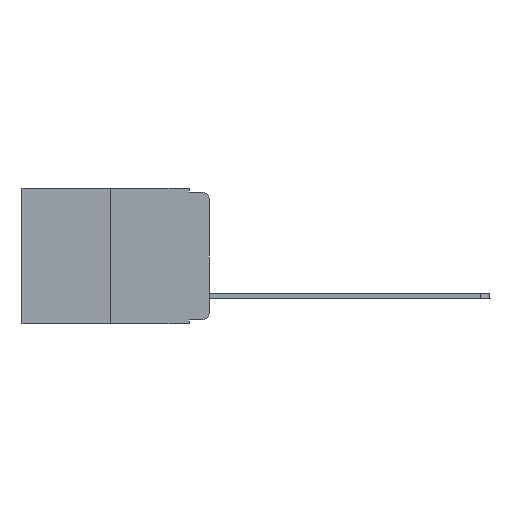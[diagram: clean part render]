
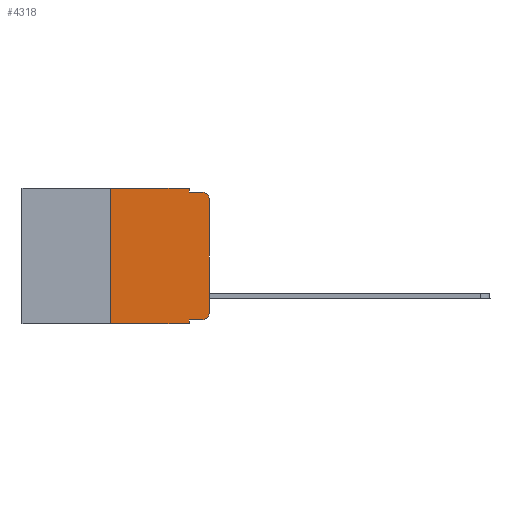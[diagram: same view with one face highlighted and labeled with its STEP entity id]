
A CAD part, left-side view. The second image highlights one B-rep face of the part: STEP entity #4318.
In plain terms, the highlighted planar face has unit normal (-1, 0, 0).
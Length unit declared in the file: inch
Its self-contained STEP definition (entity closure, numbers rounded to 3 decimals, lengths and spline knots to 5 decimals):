
#48 = CARTESIAN_POINT ( 'NONE',  ( 0., 0., 0. ) ) ;
#439 = CARTESIAN_POINT ( 'NONE',  ( 0., 0.051, -0.343 ) ) ;
#1055 = ORIENTED_EDGE ( 'NONE', *, *, #1664, .T. ) ;
#1243 = CARTESIAN_POINT ( 'NONE',  ( 0., 0.051, -0.333 ) ) ;
#1499 = DIRECTION ( 'NONE',  ( -1., 0., 0. ) ) ;
#1664 = EDGE_CURVE ( 'NONE', #16182, #15364, #4769, .T. ) ;
#1718 = ORIENTED_EDGE ( 'NONE', *, *, #10198, .T. ) ;
#1774 = VERTEX_POINT ( 'NONE', #4025 ) ;
#2221 = DIRECTION ( 'NONE',  ( -1., 0., 0. ) ) ;
#2306 = LINE ( 'NONE', #11576, #17521 ) ;
#2765 = LINE ( 'NONE', #4260, #10580 ) ;
#2769 = DIRECTION ( 'NONE',  ( 0., -1., 0. ) ) ;
#2883 = DIRECTION ( 'NONE',  ( 0., -1., 0. ) ) ;
#3223 = CARTESIAN_POINT ( 'NONE',  ( 0., 0.473, 0. ) ) ;
#3239 = ORIENTED_EDGE ( 'NONE', *, *, #17618, .F. ) ;
#3354 = PLANE ( 'NONE',  #5154 ) ;
#3363 = VERTEX_POINT ( 'NONE', #4889 ) ;
#3451 = FACE_OUTER_BOUND ( 'NONE', #11744, .T. ) ;
#3489 = DIRECTION ( 'NONE',  ( 0., -1., 0. ) ) ;
#3902 = VERTEX_POINT ( 'NONE', #439 ) ;
#4025 = CARTESIAN_POINT ( 'NONE',  ( 0., 0.051, -0.01 ) ) ;
#4229 = CARTESIAN_POINT ( 'NONE',  ( 0., 0., -0.03 ) ) ;
#4260 = CARTESIAN_POINT ( 'NONE',  ( 0., 0.25, 0. ) ) ;
#4318 = ADVANCED_FACE ( 'NONE', ( #3451 ), #3354, .F. ) ;
#4493 = LINE ( 'NONE', #7696, #18318 ) ;
#4523 = AXIS2_PLACEMENT_3D ( 'NONE', #10070, #1499, #11825 ) ;
#4549 = EDGE_CURVE ( 'NONE', #5999, #16182, #8495, .T. ) ;
#4564 = VECTOR ( 'NONE', #2883, 39.37008 ) ;
#4654 = DIRECTION ( 'NONE',  ( 0., -1., 0. ) ) ;
#4674 = DIRECTION ( 'NONE',  ( 0., 0., -1. ) ) ;
#4738 = DIRECTION ( 'NONE',  ( 0., 0., -1. ) ) ;
#4769 = CIRCLE ( 'NONE', #4523, 0.02 ) ;
#4806 = VECTOR ( 'NONE', #4738, 39.37008 ) ;
#4889 = CARTESIAN_POINT ( 'NONE',  ( 0., 0.25, 0. ) ) ;
#5154 = AXIS2_PLACEMENT_3D ( 'NONE', #3223, #9061, #4674 ) ;
#5507 = CIRCLE ( 'NONE', #7464, 0.02 ) ;
#5742 = LINE ( 'NONE', #48, #8742 ) ;
#5744 = LINE ( 'NONE', #12280, #4806 ) ;
#5773 = CARTESIAN_POINT ( 'NONE',  ( 0., 0.25, -0.343 ) ) ;
#5780 = DIRECTION ( 'NONE',  ( 0., 0., 1. ) ) ;
#5896 = ORIENTED_EDGE ( 'NONE', *, *, #4549, .T. ) ;
#5949 = VERTEX_POINT ( 'NONE', #11329 ) ;
#5999 = VERTEX_POINT ( 'NONE', #7120 ) ;
#6244 = DIRECTION ( 'NONE',  ( 0., 0., 1. ) ) ;
#6492 = CARTESIAN_POINT ( 'NONE',  ( 0., 0.473, -0.343 ) ) ;
#7046 = VECTOR ( 'NONE', #3489, 39.37008 ) ;
#7120 = CARTESIAN_POINT ( 'NONE',  ( 0., 0.051, -0.333 ) ) ;
#7332 = EDGE_CURVE ( 'NONE', #8078, #3902, #18302, .T. ) ;
#7464 = AXIS2_PLACEMENT_3D ( 'NONE', #9554, #2221, #15618 ) ;
#7696 = CARTESIAN_POINT ( 'NONE',  ( 0., 0.473, 0. ) ) ;
#8078 = VERTEX_POINT ( 'NONE', #5773 ) ;
#8189 = ORIENTED_EDGE ( 'NONE', *, *, #7332, .T. ) ;
#8495 = LINE ( 'NONE', #1243, #4564 ) ;
#8737 = VERTEX_POINT ( 'NONE', #4229 ) ;
#8742 = VECTOR ( 'NONE', #6244, 39.37008 ) ;
#9061 = DIRECTION ( 'NONE',  ( 1., 0., 0. ) ) ;
#9162 = DIRECTION ( 'NONE',  ( 0., 0., -1. ) ) ;
#9554 = CARTESIAN_POINT ( 'NONE',  ( 0., 0.02, -0.03 ) ) ;
#9882 = EDGE_CURVE ( 'NONE', #1774, #5949, #2306, .T. ) ;
#10070 = CARTESIAN_POINT ( 'NONE',  ( 0., 0.02, -0.313 ) ) ;
#10198 = EDGE_CURVE ( 'NONE', #8737, #5949, #5507, .T. ) ;
#10580 = VECTOR ( 'NONE', #5780, 39.37008 ) ;
#10931 = VECTOR ( 'NONE', #9162, 39.37008 ) ;
#11329 = CARTESIAN_POINT ( 'NONE',  ( 0., 0.02, -0.01 ) ) ;
#11576 = CARTESIAN_POINT ( 'NONE',  ( 0., 0.051, -0.01 ) ) ;
#11744 = EDGE_LOOP ( 'NONE', ( #11793, #1718, #15245, #16159, #18679, #3239, #8189, #14021, #5896, #1055 ) ) ;
#11793 = ORIENTED_EDGE ( 'NONE', *, *, #14268, .T. ) ;
#11825 = DIRECTION ( 'NONE',  ( 0., 0., -1. ) ) ;
#12280 = CARTESIAN_POINT ( 'NONE',  ( 0., 0.051, 0. ) ) ;
#14021 = ORIENTED_EDGE ( 'NONE', *, *, #17883, .F. ) ;
#14268 = EDGE_CURVE ( 'NONE', #15364, #8737, #5742, .T. ) ;
#14401 = LINE ( 'NONE', #16510, #10931 ) ;
#15245 = ORIENTED_EDGE ( 'NONE', *, *, #9882, .F. ) ;
#15364 = VERTEX_POINT ( 'NONE', #16052 ) ;
#15402 = VERTEX_POINT ( 'NONE', #17540 ) ;
#15618 = DIRECTION ( 'NONE',  ( 0., 0., -1. ) ) ;
#16052 = CARTESIAN_POINT ( 'NONE',  ( 0., 0., -0.313 ) ) ;
#16159 = ORIENTED_EDGE ( 'NONE', *, *, #16616, .F. ) ;
#16182 = VERTEX_POINT ( 'NONE', #16480 ) ;
#16480 = CARTESIAN_POINT ( 'NONE',  ( 0., 0.02, -0.333 ) ) ;
#16510 = CARTESIAN_POINT ( 'NONE',  ( 0., 0.051, 0. ) ) ;
#16616 = EDGE_CURVE ( 'NONE', #15402, #1774, #14401, .T. ) ;
#16669 = EDGE_CURVE ( 'NONE', #3363, #15402, #4493, .T. ) ;
#17521 = VECTOR ( 'NONE', #2769, 39.37008 ) ;
#17540 = CARTESIAN_POINT ( 'NONE',  ( 0., 0.051, 0. ) ) ;
#17618 = EDGE_CURVE ( 'NONE', #8078, #3363, #2765, .T. ) ;
#17883 = EDGE_CURVE ( 'NONE', #5999, #3902, #5744, .T. ) ;
#18302 = LINE ( 'NONE', #6492, #7046 ) ;
#18318 = VECTOR ( 'NONE', #4654, 39.37008 ) ;
#18679 = ORIENTED_EDGE ( 'NONE', *, *, #16669, .F. ) ;
